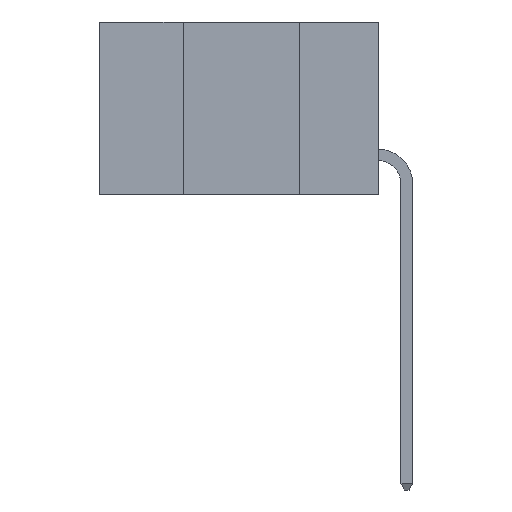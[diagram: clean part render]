
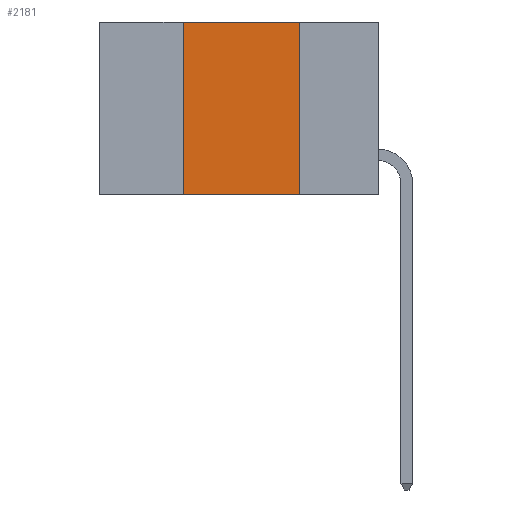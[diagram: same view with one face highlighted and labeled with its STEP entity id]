
A CAD part, left-side view. The second image highlights one B-rep face of the part: STEP entity #2181.
In plain terms, the highlighted planar face has unit normal (-1, 0, 0).
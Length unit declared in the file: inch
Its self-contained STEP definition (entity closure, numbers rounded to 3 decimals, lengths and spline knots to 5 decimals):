
#316 = DIRECTION ( 'NONE',  ( 0., 0., -1. ) ) ;
#1283 = DIRECTION ( 'NONE',  ( 1., 0., 0. ) ) ;
#1413 = PLANE ( 'NONE',  #12410 ) ;
#2181 = ADVANCED_FACE ( 'NONE', ( #14934 ), #1413, .F. ) ;
#2536 = CARTESIAN_POINT ( 'NONE',  ( 0., 0.17, 0. ) ) ;
#2573 = CARTESIAN_POINT ( 'NONE',  ( 0., 0.17, -0.37 ) ) ;
#2901 = ORIENTED_EDGE ( 'NONE', *, *, #14594, .T. ) ;
#4030 = VECTOR ( 'NONE', #316, 39.37008 ) ;
#4468 = ORIENTED_EDGE ( 'NONE', *, *, #24257, .F. ) ;
#4665 = LINE ( 'NONE', #14137, #4030 ) ;
#5999 = ORIENTED_EDGE ( 'NONE', *, *, #8455, .F. ) ;
#6426 = CARTESIAN_POINT ( 'NONE',  ( 0., 0.42, -0.37 ) ) ;
#6588 = VECTOR ( 'NONE', #13231, 39.37008 ) ;
#7748 = VECTOR ( 'NONE', #8436, 39.37008 ) ;
#8436 = DIRECTION ( 'NONE',  ( 0., 0., 1. ) ) ;
#8455 = EDGE_CURVE ( 'NONE', #20966, #10866, #4665, .T. ) ;
#8925 = EDGE_CURVE ( 'NONE', #18566, #20966, #19700, .T. ) ;
#10836 = VERTEX_POINT ( 'NONE', #6426 ) ;
#10866 = VERTEX_POINT ( 'NONE', #2573 ) ;
#11245 = DIRECTION ( 'NONE',  ( 0., 0., -1. ) ) ;
#12410 = AXIS2_PLACEMENT_3D ( 'NONE', #15953, #1283, #11245 ) ;
#12988 = LINE ( 'NONE', #16264, #7748 ) ;
#13231 = DIRECTION ( 'NONE',  ( 0., -1., 0. ) ) ;
#14137 = CARTESIAN_POINT ( 'NONE',  ( 0., 0.17, -0.37 ) ) ;
#14594 = EDGE_CURVE ( 'NONE', #10836, #10866, #16413, .T. ) ;
#14934 = FACE_OUTER_BOUND ( 'NONE', #25058, .T. ) ;
#15953 = CARTESIAN_POINT ( 'NONE',  ( 0., 0.6, 0. ) ) ;
#16264 = CARTESIAN_POINT ( 'NONE',  ( 0., 0.42, -0.37 ) ) ;
#16413 = LINE ( 'NONE', #24951, #6588 ) ;
#17631 = DIRECTION ( 'NONE',  ( 0., -1., 0. ) ) ;
#17976 = ORIENTED_EDGE ( 'NONE', *, *, #8925, .F. ) ;
#18566 = VERTEX_POINT ( 'NONE', #19181 ) ;
#19096 = VECTOR ( 'NONE', #17631, 39.37008 ) ;
#19181 = CARTESIAN_POINT ( 'NONE',  ( 0., 0.42, 0. ) ) ;
#19700 = LINE ( 'NONE', #25491, #19096 ) ;
#20966 = VERTEX_POINT ( 'NONE', #2536 ) ;
#24257 = EDGE_CURVE ( 'NONE', #10836, #18566, #12988, .T. ) ;
#24951 = CARTESIAN_POINT ( 'NONE',  ( 0., 0.6, -0.37 ) ) ;
#25058 = EDGE_LOOP ( 'NONE', ( #5999, #17976, #4468, #2901 ) ) ;
#25491 = CARTESIAN_POINT ( 'NONE',  ( 0., 0.6, 0. ) ) ;
